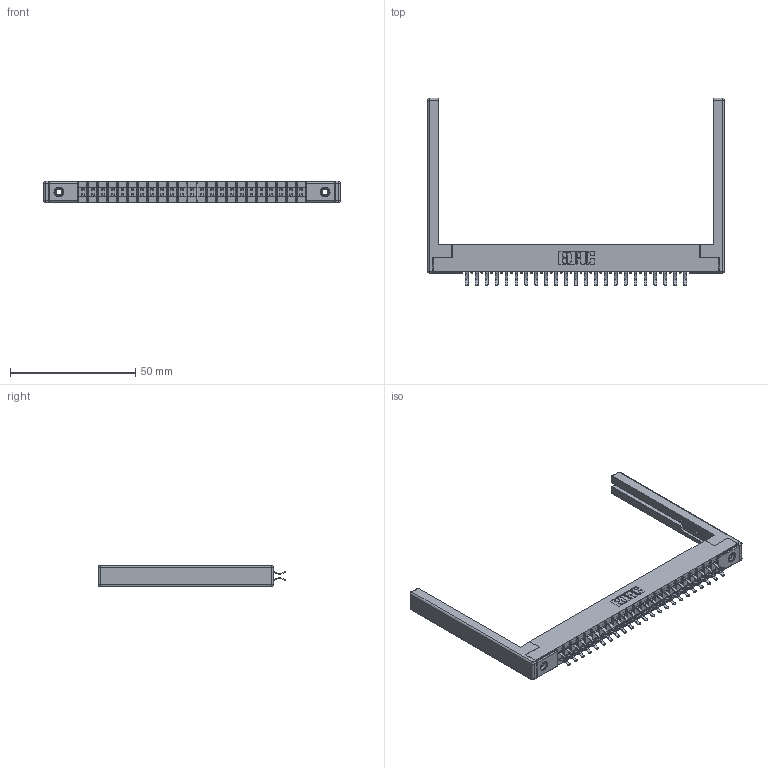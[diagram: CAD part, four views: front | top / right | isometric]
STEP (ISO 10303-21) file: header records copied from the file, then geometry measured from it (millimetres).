
FILE_DESCRIPTION (( 'STEP AP203' ), '1' );
FILE_NAME ('355-046-556-568.STEP', '2019-09-11T15:00:15', ( '' ), ( '' ), 'SwSTEP 2.0', 'SolidWorks 2016', '' );
FILE_SCHEMA (( 'CONFIG_CONTROL_DESIGN' ));
Length unit declared in the file: inch
Products named in the file (5): 355-046-556-568; 305-290-001_556; 307-220-068; 305 Part_.156 Dia; 345-250-001_345-250-001-102
Assembly tree (51 placements, depth 2):
  355-046-556-568
    305 Part_.156 Dia
    305-290-001_556  x46
    345-250-001_345-250-001-102  x2
    307-220-068  x2
Bounding box: 118.57 x 74.93 x 8.71 mm (x, y, z)
Volume: 11679.9 mm3; surface area: 18242.8 mm2
Topology: 51 solids, 51 shells, 2846 faces, 8135 edges, 5278 vertices
Faces by surface type: plane 1582, cylinder 1148, sphere 100, cone 12, torus 4
Entity records: 30197 total; most frequent: CARTESIAN_POINT 4972, ORIENTED_EDGE 4924, DIRECTION 4848, EDGE_CURVE 2462, LINE 1956, VECTOR 1956, VERTEX_POINT 1570, AXIS2_PLACEMENT_3D 1446
